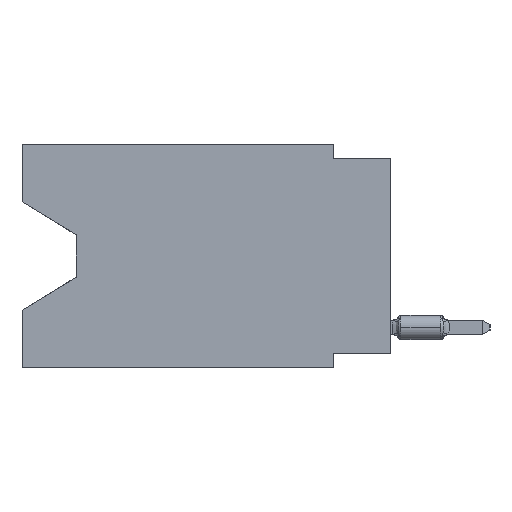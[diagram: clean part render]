
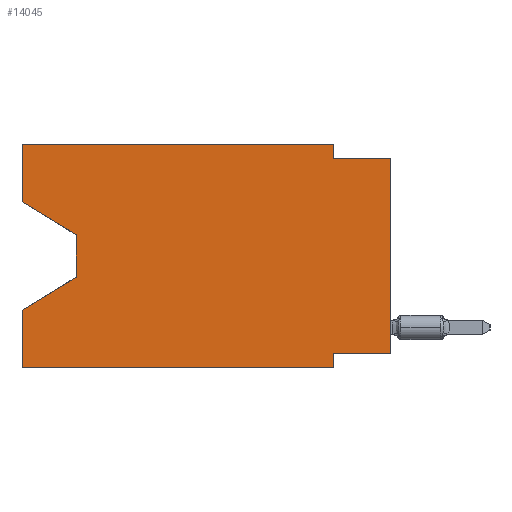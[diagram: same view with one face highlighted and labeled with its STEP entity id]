
A CAD part, left-side view. The second image highlights one B-rep face of the part: STEP entity #14045.
In plain terms, the highlighted planar face has unit normal (-1, 0, 0).
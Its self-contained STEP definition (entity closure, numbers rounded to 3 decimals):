
#110 = VECTOR ( 'NONE', #5977, 1000. ) ;
#901 = DIRECTION ( 'NONE',  ( 0., 0., -1. ) ) ;
#1357 = VECTOR ( 'NONE', #37790, 1000. ) ;
#1842 = VECTOR ( 'NONE', #45053, 1000. ) ;
#3082 = DIRECTION ( 'NONE',  ( 1., 0., 0. ) ) ;
#3505 = VERTEX_POINT ( 'NONE', #20563 ) ;
#3714 = CARTESIAN_POINT ( 'NONE',  ( 0., 0., 0. ) ) ;
#4015 = VERTEX_POINT ( 'NONE', #11411 ) ;
#5977 = DIRECTION ( 'NONE',  ( 0., -1., 0. ) ) ;
#6641 = VERTEX_POINT ( 'NONE', #26832 ) ;
#6869 = LINE ( 'NONE', #17502, #36153 ) ;
#7353 = AXIS2_PLACEMENT_3D ( 'NONE', #13228, #3082, #27767 ) ;
#8730 = LINE ( 'NONE', #19369, #110 ) ;
#8836 = VECTOR ( 'NONE', #13389, 1000. ) ;
#8878 = EDGE_CURVE ( 'NONE', #10980, #39966, #10070, .T. ) ;
#9296 = DIRECTION ( 'NONE',  ( 0., 0., 1. ) ) ;
#9715 = EDGE_CURVE ( 'NONE', #10980, #3505, #6869, .T. ) ;
#9778 = VERTEX_POINT ( 'NONE', #15187 ) ;
#9903 = LINE ( 'NONE', #14061, #8836 ) ;
#10070 = LINE ( 'NONE', #35513, #15395 ) ;
#10588 = EDGE_CURVE ( 'NONE', #45235, #30951, #39127, .T. ) ;
#10980 = VERTEX_POINT ( 'NONE', #21902 ) ;
#11411 = CARTESIAN_POINT ( 'NONE',  ( 0., 16.383, -7.36 ) ) ;
#11414 = EDGE_CURVE ( 'NONE', #39966, #45235, #15367, .T. ) ;
#11829 = VERTEX_POINT ( 'NONE', #15998 ) ;
#11961 = ORIENTED_EDGE ( 'NONE', *, *, #25111, .T. ) ;
#13228 = CARTESIAN_POINT ( 'NONE',  ( 0., 16.383, 0. ) ) ;
#13389 = DIRECTION ( 'NONE',  ( 0., 0.855, -0.519 ) ) ;
#14045 = ADVANCED_FACE ( 'NONE', ( #23866 ), #37965, .F. ) ;
#14061 = CARTESIAN_POINT ( 'NONE',  ( 0., 13.97, -5.893 ) ) ;
#14284 = LINE ( 'NONE', #27921, #37400 ) ;
#14370 = CARTESIAN_POINT ( 'NONE',  ( 0., 2.54, 0. ) ) ;
#15187 = CARTESIAN_POINT ( 'NONE',  ( 0., 2.54, -9.906 ) ) ;
#15367 = LINE ( 'NONE', #23212, #21459 ) ;
#15395 = VECTOR ( 'NONE', #24625, 1000. ) ;
#15875 = EDGE_CURVE ( 'NONE', #37181, #19091, #17309, .T. ) ;
#15986 = EDGE_CURVE ( 'NONE', #11829, #9778, #8730, .T. ) ;
#15998 = CARTESIAN_POINT ( 'NONE',  ( 0., 16.383, -9.906 ) ) ;
#16627 = ORIENTED_EDGE ( 'NONE', *, *, #15875, .T. ) ;
#16701 = VECTOR ( 'NONE', #901, 1000. ) ;
#17309 = LINE ( 'NONE', #3714, #42939 ) ;
#17502 = CARTESIAN_POINT ( 'NONE',  ( 0., 16.383, -2.546 ) ) ;
#17835 = ORIENTED_EDGE ( 'NONE', *, *, #9715, .T. ) ;
#18149 = CARTESIAN_POINT ( 'NONE',  ( 0., 2.54, -0.635 ) ) ;
#18466 = ORIENTED_EDGE ( 'NONE', *, *, #29975, .F. ) ;
#18865 = DIRECTION ( 'NONE',  ( 0., 0., -1. ) ) ;
#18903 = EDGE_CURVE ( 'NONE', #3505, #32232, #39942, .T. ) ;
#19091 = VERTEX_POINT ( 'NONE', #30442 ) ;
#19369 = CARTESIAN_POINT ( 'NONE',  ( 0., 16.383, -9.906 ) ) ;
#20563 = CARTESIAN_POINT ( 'NONE',  ( 0., 13.97, -4.013 ) ) ;
#21459 = VECTOR ( 'NONE', #33848, 1000. ) ;
#21902 = CARTESIAN_POINT ( 'NONE',  ( 0., 16.383, -2.546 ) ) ;
#23212 = CARTESIAN_POINT ( 'NONE',  ( 0., 16.383, 0. ) ) ;
#23866 = FACE_OUTER_BOUND ( 'NONE', #45314, .T. ) ;
#24465 = DIRECTION ( 'NONE',  ( 0., 1., 0. ) ) ;
#24625 = DIRECTION ( 'NONE',  ( 0., 0., 1. ) ) ;
#24917 = ORIENTED_EDGE ( 'NONE', *, *, #10588, .F. ) ;
#25111 = EDGE_CURVE ( 'NONE', #32232, #4015, #9903, .T. ) ;
#25166 = EDGE_CURVE ( 'NONE', #37181, #6641, #14284, .T. ) ;
#25366 = CARTESIAN_POINT ( 'NONE',  ( 0., 13.97, -4.013 ) ) ;
#25927 = VECTOR ( 'NONE', #18865, 1000. ) ;
#26832 = CARTESIAN_POINT ( 'NONE',  ( 0., 2.54, -9.271 ) ) ;
#26926 = EDGE_CURVE ( 'NONE', #30951, #19091, #35209, .T. ) ;
#27685 = CARTESIAN_POINT ( 'NONE',  ( 0., 16.383, 0. ) ) ;
#27767 = DIRECTION ( 'NONE',  ( 0., 0., -1. ) ) ;
#27921 = CARTESIAN_POINT ( 'NONE',  ( 0., 0., -9.271 ) ) ;
#28084 = ORIENTED_EDGE ( 'NONE', *, *, #44523, .F. ) ;
#28484 = DIRECTION ( 'NONE',  ( 0., 0., -1. ) ) ;
#28684 = ORIENTED_EDGE ( 'NONE', *, *, #26926, .F. ) ;
#28838 = CARTESIAN_POINT ( 'NONE',  ( 0., 0., -9.271 ) ) ;
#29285 = LINE ( 'NONE', #43383, #25927 ) ;
#29975 = EDGE_CURVE ( 'NONE', #11829, #4015, #44821, .T. ) ;
#30039 = ORIENTED_EDGE ( 'NONE', *, *, #15986, .T. ) ;
#30442 = CARTESIAN_POINT ( 'NONE',  ( 0., 0., -0.635 ) ) ;
#30951 = VERTEX_POINT ( 'NONE', #18149 ) ;
#32232 = VERTEX_POINT ( 'NONE', #36628 ) ;
#33280 = ORIENTED_EDGE ( 'NONE', *, *, #18903, .T. ) ;
#33848 = DIRECTION ( 'NONE',  ( 0., -1., 0. ) ) ;
#34628 = DIRECTION ( 'NONE',  ( 0., -0.855, -0.519 ) ) ;
#35209 = LINE ( 'NONE', #41264, #1357 ) ;
#35415 = VECTOR ( 'NONE', #28484, 1000. ) ;
#35513 = CARTESIAN_POINT ( 'NONE',  ( 0., 16.383, 0. ) ) ;
#36153 = VECTOR ( 'NONE', #34628, 1000. ) ;
#36628 = CARTESIAN_POINT ( 'NONE',  ( 0., 13.97, -5.893 ) ) ;
#37181 = VERTEX_POINT ( 'NONE', #28838 ) ;
#37400 = VECTOR ( 'NONE', #24465, 1000. ) ;
#37790 = DIRECTION ( 'NONE',  ( 0., -1., 0. ) ) ;
#37965 = PLANE ( 'NONE',  #7353 ) ;
#38096 = CARTESIAN_POINT ( 'NONE',  ( 0., 16.383, 0. ) ) ;
#39127 = LINE ( 'NONE', #14370, #35415 ) ;
#39942 = LINE ( 'NONE', #25366, #16701 ) ;
#39966 = VERTEX_POINT ( 'NONE', #38096 ) ;
#41264 = CARTESIAN_POINT ( 'NONE',  ( 0., 0., -0.635 ) ) ;
#42389 = ORIENTED_EDGE ( 'NONE', *, *, #8878, .F. ) ;
#42939 = VECTOR ( 'NONE', #9296, 1000. ) ;
#43383 = CARTESIAN_POINT ( 'NONE',  ( 0., 2.54, -9.906 ) ) ;
#43829 = ORIENTED_EDGE ( 'NONE', *, *, #11414, .F. ) ;
#43883 = CARTESIAN_POINT ( 'NONE',  ( 0., 2.54, 0. ) ) ;
#44523 = EDGE_CURVE ( 'NONE', #6641, #9778, #29285, .T. ) ;
#44821 = LINE ( 'NONE', #27685, #1842 ) ;
#45053 = DIRECTION ( 'NONE',  ( 0., 0., 1. ) ) ;
#45235 = VERTEX_POINT ( 'NONE', #43883 ) ;
#45314 = EDGE_LOOP ( 'NONE', ( #17835, #33280, #11961, #18466, #30039, #28084, #45545, #16627, #28684, #24917, #43829, #42389 ) ) ;
#45545 = ORIENTED_EDGE ( 'NONE', *, *, #25166, .F. ) ;
